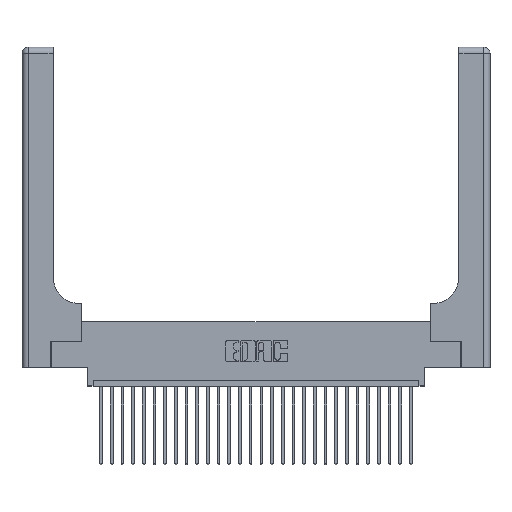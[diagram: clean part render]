
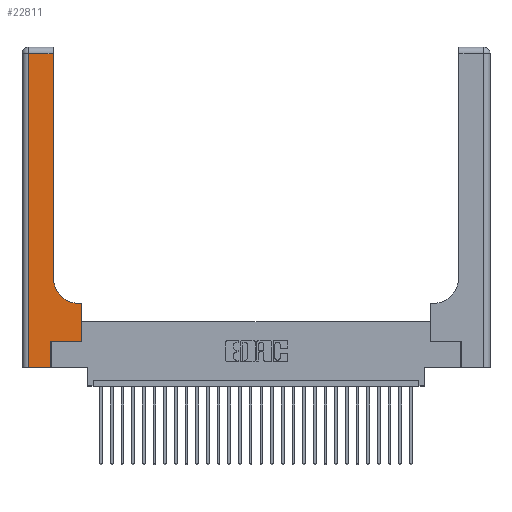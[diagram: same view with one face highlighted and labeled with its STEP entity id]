
A CAD part, top view. The second image highlights one B-rep face of the part: STEP entity #22811.
In plain terms, the highlighted planar face has unit normal (0, 0, 1).
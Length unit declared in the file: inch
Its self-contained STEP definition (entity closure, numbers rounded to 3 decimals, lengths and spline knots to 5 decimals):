
#75 = ORIENTED_EDGE ( 'NONE', *, *, #16550, .T. ) ;
#361 = DIRECTION ( 'NONE',  ( 1., 0., 0. ) ) ;
#400 = CARTESIAN_POINT ( 'NONE',  ( 0.2915, 2.94, 0.37 ) ) ;
#765 = VECTOR ( 'NONE', #18639, 39.37008 ) ;
#1006 = EDGE_CURVE ( 'NONE', #3889, #6500, #28992, .T. ) ;
#1279 = EDGE_CURVE ( 'NONE', #23084, #6954, #5805, .T. ) ;
#1729 = DIRECTION ( 'NONE',  ( 0., -1., 0. ) ) ;
#2449 = VERTEX_POINT ( 'NONE', #400 ) ;
#2818 = VECTOR ( 'NONE', #14432, 39.37008 ) ;
#3153 = AXIS2_PLACEMENT_3D ( 'NONE', #6318, #26947, #24619 ) ;
#3566 = ORIENTED_EDGE ( 'NONE', *, *, #1006, .T. ) ;
#3889 = VERTEX_POINT ( 'NONE', #5531 ) ;
#4266 = VECTOR ( 'NONE', #21879, 39.37008 ) ;
#4627 = CARTESIAN_POINT ( 'NONE',  ( 0.5585, 0.6, 0.37 ) ) ;
#4682 = VERTEX_POINT ( 'NONE', #11365 ) ;
#5181 = VERTEX_POINT ( 'NONE', #25885 ) ;
#5531 = CARTESIAN_POINT ( 'NONE',  ( 0.5585, 0.25, 0.37 ) ) ;
#5805 = LINE ( 'NONE', #15951, #12564 ) ;
#6318 = CARTESIAN_POINT ( 'NONE',  ( 0., 3., 0.37 ) ) ;
#6362 = ORIENTED_EDGE ( 'NONE', *, *, #13594, .T. ) ;
#6367 = ORIENTED_EDGE ( 'NONE', *, *, #19007, .T. ) ;
#6500 = VERTEX_POINT ( 'NONE', #4627 ) ;
#6873 = VECTOR ( 'NONE', #26011, 39.37008 ) ;
#6954 = VERTEX_POINT ( 'NONE', #7547 ) ;
#6976 = CARTESIAN_POINT ( 'NONE',  ( 0.2915, 0.6, 0.37 ) ) ;
#7031 = LINE ( 'NONE', #15423, #12050 ) ;
#7377 = LINE ( 'NONE', #23591, #10603 ) ;
#7547 = CARTESIAN_POINT ( 'NONE',  ( 0.269, 0., 0.37 ) ) ;
#8479 = ORIENTED_EDGE ( 'NONE', *, *, #1279, .T. ) ;
#9559 = CARTESIAN_POINT ( 'NONE',  ( 0.269, 0.25, 0.37 ) ) ;
#10327 = LINE ( 'NONE', #17286, #4266 ) ;
#10603 = VECTOR ( 'NONE', #28408, 39.37008 ) ;
#11267 = VERTEX_POINT ( 'NONE', #9559 ) ;
#11328 = ORIENTED_EDGE ( 'NONE', *, *, #18304, .T. ) ;
#11365 = CARTESIAN_POINT ( 'NONE',  ( 0.06, 2.94, 0.37 ) ) ;
#12050 = VECTOR ( 'NONE', #20253, 39.37008 ) ;
#12355 = FACE_OUTER_BOUND ( 'NONE', #23715, .T. ) ;
#12564 = VECTOR ( 'NONE', #361, 39.37008 ) ;
#13594 = EDGE_CURVE ( 'NONE', #2449, #4682, #10327, .T. ) ;
#14432 = DIRECTION ( 'NONE',  ( 0., 1., 0. ) ) ;
#15384 = CARTESIAN_POINT ( 'NONE',  ( 0.06, 3., 0.37 ) ) ;
#15423 = CARTESIAN_POINT ( 'NONE',  ( 0.269, 0., 0.37 ) ) ;
#15951 = CARTESIAN_POINT ( 'NONE',  ( 0., 0., 0.37 ) ) ;
#16090 = AXIS2_PLACEMENT_3D ( 'NONE', #28860, #28555, #21995 ) ;
#16373 = LINE ( 'NONE', #27971, #2818 ) ;
#16550 = EDGE_CURVE ( 'NONE', #4682, #23084, #28730, .T. ) ;
#17286 = CARTESIAN_POINT ( 'NONE',  ( 0., 2.94, 0.37 ) ) ;
#18304 = EDGE_CURVE ( 'NONE', #5181, #25755, #19342, .T. ) ;
#18401 = ORIENTED_EDGE ( 'NONE', *, *, #21000, .T. ) ;
#18639 = DIRECTION ( 'NONE',  ( -1., 0., 0. ) ) ;
#19007 = EDGE_CURVE ( 'NONE', #6500, #5181, #21809, .T. ) ;
#19342 = CIRCLE ( 'NONE', #16090, 0.25 ) ;
#20238 = EDGE_CURVE ( 'NONE', #25755, #2449, #16373, .T. ) ;
#20253 = DIRECTION ( 'NONE',  ( 0., 1., 0. ) ) ;
#21000 = EDGE_CURVE ( 'NONE', #6954, #11267, #7031, .T. ) ;
#21015 = CARTESIAN_POINT ( 'NONE',  ( 0.06, 0., 0.37 ) ) ;
#21045 = ORIENTED_EDGE ( 'NONE', *, *, #21321, .T. ) ;
#21321 = EDGE_CURVE ( 'NONE', #11267, #3889, #7377, .T. ) ;
#21715 = CARTESIAN_POINT ( 'NONE',  ( 0.2915, 0.85, 0.37 ) ) ;
#21809 = LINE ( 'NONE', #6976, #765 ) ;
#21879 = DIRECTION ( 'NONE',  ( -1., 0., 0. ) ) ;
#21995 = DIRECTION ( 'NONE',  ( 1., 0., 0. ) ) ;
#22811 = ADVANCED_FACE ( 'NONE', ( #12355 ), #24431, .F. ) ;
#23084 = VERTEX_POINT ( 'NONE', #21015 ) ;
#23591 = CARTESIAN_POINT ( 'NONE',  ( 0.269, 0.25, 0.37 ) ) ;
#23715 = EDGE_LOOP ( 'NONE', ( #26270, #6362, #75, #8479, #18401, #21045, #3566, #6367, #11328 ) ) ;
#24431 = PLANE ( 'NONE',  #3153 ) ;
#24619 = DIRECTION ( 'NONE',  ( -1., 0., 0. ) ) ;
#25492 = VECTOR ( 'NONE', #1729, 39.37008 ) ;
#25755 = VERTEX_POINT ( 'NONE', #21715 ) ;
#25885 = CARTESIAN_POINT ( 'NONE',  ( 0.5415, 0.6, 0.37 ) ) ;
#26011 = DIRECTION ( 'NONE',  ( 0., 1., 0. ) ) ;
#26270 = ORIENTED_EDGE ( 'NONE', *, *, #20238, .T. ) ;
#26947 = DIRECTION ( 'NONE',  ( 0., 0., -1. ) ) ;
#27971 = CARTESIAN_POINT ( 'NONE',  ( 0.2915, 3., 0.37 ) ) ;
#28211 = CARTESIAN_POINT ( 'NONE',  ( 0.5585, 0.25, 0.37 ) ) ;
#28408 = DIRECTION ( 'NONE',  ( 1., 0., 0. ) ) ;
#28555 = DIRECTION ( 'NONE',  ( 0., 0., -1. ) ) ;
#28730 = LINE ( 'NONE', #15384, #25492 ) ;
#28860 = CARTESIAN_POINT ( 'NONE',  ( 0.5415, 0.85, 0.37 ) ) ;
#28992 = LINE ( 'NONE', #28211, #6873 ) ;
